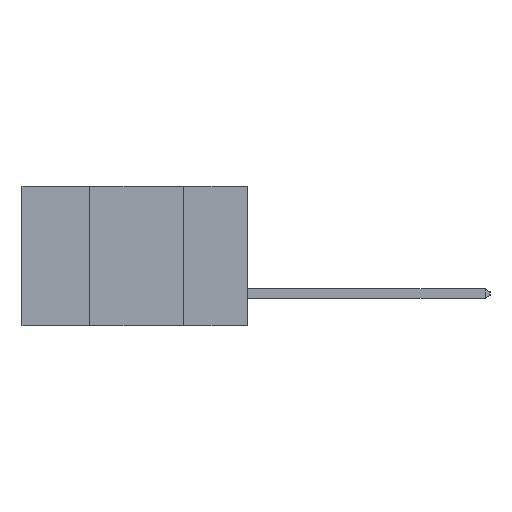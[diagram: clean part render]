
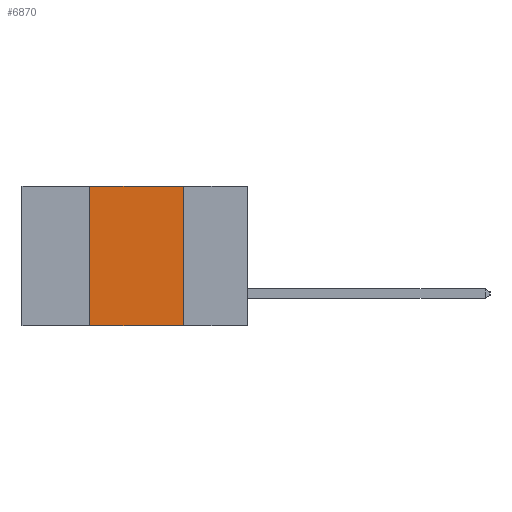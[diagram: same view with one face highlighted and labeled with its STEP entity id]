
A CAD part, left-side view. The second image highlights one B-rep face of the part: STEP entity #6870.
In plain terms, the highlighted planar face has unit normal (-1, 0, 0).
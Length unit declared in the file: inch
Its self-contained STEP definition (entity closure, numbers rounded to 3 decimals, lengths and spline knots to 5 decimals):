
#596 = ORIENTED_EDGE ( 'NONE', *, *, #9571, .F. ) ;
#833 = CARTESIAN_POINT ( 'NONE',  ( 0., 0.17, -0.37 ) ) ;
#1939 = ORIENTED_EDGE ( 'NONE', *, *, #7416, .T. ) ;
#2231 = DIRECTION ( 'NONE',  ( 0., 0., 1. ) ) ;
#2544 = VERTEX_POINT ( 'NONE', #9550 ) ;
#2710 = DIRECTION ( 'NONE',  ( 0., 0., -1. ) ) ;
#2764 = DIRECTION ( 'NONE',  ( 1., 0., 0. ) ) ;
#2887 = PLANE ( 'NONE',  #6065 ) ;
#2969 = DIRECTION ( 'NONE',  ( 0., 0., -1. ) ) ;
#3601 = ORIENTED_EDGE ( 'NONE', *, *, #20177, .F. ) ;
#3873 = CARTESIAN_POINT ( 'NONE',  ( 0., 0.6, 0. ) ) ;
#4778 = VECTOR ( 'NONE', #2231, 39.37008 ) ;
#5608 = LINE ( 'NONE', #7946, #25789 ) ;
#5810 = VERTEX_POINT ( 'NONE', #15791 ) ;
#5862 = VERTEX_POINT ( 'NONE', #12459 ) ;
#6065 = AXIS2_PLACEMENT_3D ( 'NONE', #3873, #2764, #2710 ) ;
#6764 = DIRECTION ( 'NONE',  ( 0., -1., 0. ) ) ;
#6870 = ADVANCED_FACE ( 'NONE', ( #7091 ), #2887, .F. ) ;
#7049 = ORIENTED_EDGE ( 'NONE', *, *, #13663, .F. ) ;
#7091 = FACE_OUTER_BOUND ( 'NONE', #13794, .T. ) ;
#7416 = EDGE_CURVE ( 'NONE', #5862, #2544, #8665, .T. ) ;
#7946 = CARTESIAN_POINT ( 'NONE',  ( 0., 0.6, 0. ) ) ;
#8011 = VECTOR ( 'NONE', #12900, 39.37008 ) ;
#8368 = CARTESIAN_POINT ( 'NONE',  ( 0., 0.42, -0.37 ) ) ;
#8665 = LINE ( 'NONE', #13806, #8011 ) ;
#9550 = CARTESIAN_POINT ( 'NONE',  ( 0., 0.17, -0.37 ) ) ;
#9571 = EDGE_CURVE ( 'NONE', #5810, #20521, #5608, .T. ) ;
#12459 = CARTESIAN_POINT ( 'NONE',  ( 0., 0.42, -0.37 ) ) ;
#12900 = DIRECTION ( 'NONE',  ( 0., -1., 0. ) ) ;
#13663 = EDGE_CURVE ( 'NONE', #20521, #2544, #26092, .T. ) ;
#13794 = EDGE_LOOP ( 'NONE', ( #7049, #596, #3601, #1939 ) ) ;
#13806 = CARTESIAN_POINT ( 'NONE',  ( 0., 0.6, -0.37 ) ) ;
#15791 = CARTESIAN_POINT ( 'NONE',  ( 0., 0.42, 0. ) ) ;
#20177 = EDGE_CURVE ( 'NONE', #5862, #5810, #21592, .T. ) ;
#20521 = VERTEX_POINT ( 'NONE', #21610 ) ;
#20880 = VECTOR ( 'NONE', #2969, 39.37008 ) ;
#21592 = LINE ( 'NONE', #8368, #4778 ) ;
#21610 = CARTESIAN_POINT ( 'NONE',  ( 0., 0.17, 0. ) ) ;
#25789 = VECTOR ( 'NONE', #6764, 39.37008 ) ;
#26092 = LINE ( 'NONE', #833, #20880 ) ;
